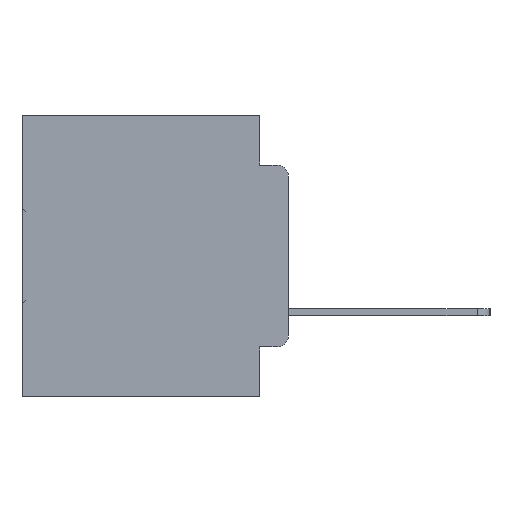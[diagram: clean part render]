
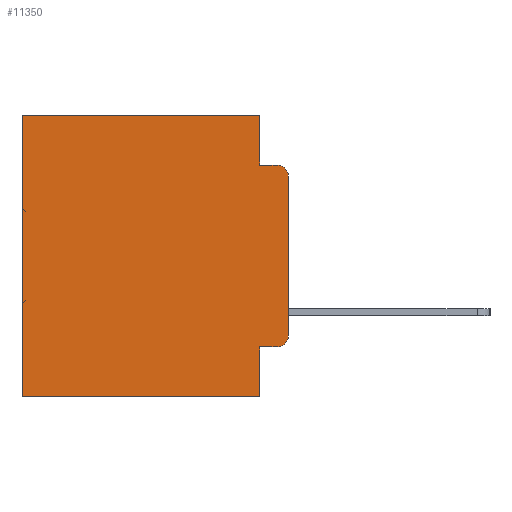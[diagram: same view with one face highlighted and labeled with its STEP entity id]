
A CAD part, left-side view. The second image highlights one B-rep face of the part: STEP entity #11350.
In plain terms, the highlighted planar face has unit normal (-1, 0, 0).
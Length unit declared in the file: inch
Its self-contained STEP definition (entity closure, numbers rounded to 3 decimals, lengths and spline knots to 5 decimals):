
#225 = VERTEX_POINT ( 'NONE', #13336 ) ;
#260 = CARTESIAN_POINT ( 'NONE',  ( 0.298, 0.02, -0.3915 ) ) ;
#282 = CARTESIAN_POINT ( 'NONE',  ( 0.298, 0.051, -0.4115 ) ) ;
#612 = VERTEX_POINT ( 'NONE', #30780 ) ;
#1627 = EDGE_CURVE ( 'NONE', #612, #17676, #18233, .T. ) ;
#1870 = DIRECTION ( 'NONE',  ( 0., -1., 0. ) ) ;
#1932 = CARTESIAN_POINT ( 'NONE',  ( 0.298, 0., 0. ) ) ;
#2597 = LINE ( 'NONE', #282, #29986 ) ;
#2846 = DIRECTION ( 'NONE',  ( 0., 0., -1. ) ) ;
#3049 = VECTOR ( 'NONE', #9485, 39.37008 ) ;
#3264 = LINE ( 'NONE', #29891, #16380 ) ;
#3346 = EDGE_CURVE ( 'NONE', #28680, #26283, #18556, .T. ) ;
#3871 = VECTOR ( 'NONE', #1870, 39.37008 ) ;
#4135 = DIRECTION ( 'NONE',  ( 0., 1., 0. ) ) ;
#4545 = DIRECTION ( 'NONE',  ( 0., 0., -1. ) ) ;
#4864 = VERTEX_POINT ( 'NONE', #20870 ) ;
#5791 = EDGE_CURVE ( 'NONE', #4864, #17000, #7734, .T. ) ;
#6125 = ORIENTED_EDGE ( 'NONE', *, *, #3346, .F. ) ;
#6180 = DIRECTION ( 'NONE',  ( 0., 1., 0. ) ) ;
#6495 = ORIENTED_EDGE ( 'NONE', *, *, #25176, .T. ) ;
#7278 = ORIENTED_EDGE ( 'NONE', *, *, #24792, .F. ) ;
#7734 = LINE ( 'NONE', #29913, #13092 ) ;
#8023 = DIRECTION ( 'NONE',  ( 0., 0., -1. ) ) ;
#8665 = EDGE_CURVE ( 'NONE', #28680, #31448, #2597, .T. ) ;
#9188 = CARTESIAN_POINT ( 'NONE',  ( 0.298, 0.051, 0. ) ) ;
#9239 = LINE ( 'NONE', #24396, #3049 ) ;
#9485 = DIRECTION ( 'NONE',  ( 0., 0., -1. ) ) ;
#10274 = DIRECTION ( 'NONE',  ( -1., 0., 0. ) ) ;
#11350 = ADVANCED_FACE ( 'NONE', ( #23594 ), #17555, .F. ) ;
#12022 = AXIS2_PLACEMENT_3D ( 'NONE', #260, #18476, #2846 ) ;
#12406 = EDGE_CURVE ( 'NONE', #26283, #17676, #3264, .T. ) ;
#12514 = VECTOR ( 'NONE', #6180, 39.37008 ) ;
#13092 = VECTOR ( 'NONE', #22371, 39.37008 ) ;
#13336 = CARTESIAN_POINT ( 'NONE',  ( 0.298, 0.051, -0.0885 ) ) ;
#13847 = ORIENTED_EDGE ( 'NONE', *, *, #23095, .T. ) ;
#13933 = EDGE_CURVE ( 'NONE', #31448, #17000, #23408, .T. ) ;
#14462 = CARTESIAN_POINT ( 'NONE',  ( 0.298, 0.02, -0.4115 ) ) ;
#15552 = ORIENTED_EDGE ( 'NONE', *, *, #8665, .T. ) ;
#16380 = VECTOR ( 'NONE', #4135, 39.37008 ) ;
#17000 = VERTEX_POINT ( 'NONE', #20165 ) ;
#17353 = VERTEX_POINT ( 'NONE', #26588 ) ;
#17500 = VERTEX_POINT ( 'NONE', #24589 ) ;
#17555 = PLANE ( 'NONE',  #24556 ) ;
#17676 = VERTEX_POINT ( 'NONE', #20352 ) ;
#17770 = LINE ( 'NONE', #27684, #3871 ) ;
#18233 = LINE ( 'NONE', #31635, #22556 ) ;
#18476 = DIRECTION ( 'NONE',  ( -1., 0., 0. ) ) ;
#18498 = DIRECTION ( 'NONE',  ( 0., -1., 0. ) ) ;
#18556 = LINE ( 'NONE', #9188, #31191 ) ;
#19328 = LINE ( 'NONE', #21649, #12514 ) ;
#19863 = ORIENTED_EDGE ( 'NONE', *, *, #29887, .F. ) ;
#20085 = DIRECTION ( 'NONE',  ( 1., 0., 0. ) ) ;
#20165 = CARTESIAN_POINT ( 'NONE',  ( 0.298, 0., -0.3915 ) ) ;
#20352 = CARTESIAN_POINT ( 'NONE',  ( 0.298, 0.473, -0.5 ) ) ;
#20361 = ORIENTED_EDGE ( 'NONE', *, *, #13933, .T. ) ;
#20551 = EDGE_LOOP ( 'NONE', ( #30861, #13847, #7278, #19863, #6495, #20680, #25438, #6125, #15552, #20361 ) ) ;
#20680 = ORIENTED_EDGE ( 'NONE', *, *, #1627, .T. ) ;
#20870 = CARTESIAN_POINT ( 'NONE',  ( 0.298, 0., -0.1085 ) ) ;
#21586 = CARTESIAN_POINT ( 'NONE',  ( 0.298, 0.051, -0.5 ) ) ;
#21649 = CARTESIAN_POINT ( 'NONE',  ( 0.298, 0., 0. ) ) ;
#22371 = DIRECTION ( 'NONE',  ( 0., 0., -1. ) ) ;
#22556 = VECTOR ( 'NONE', #27065, 39.37008 ) ;
#23095 = EDGE_CURVE ( 'NONE', #4864, #17500, #29335, .T. ) ;
#23408 = CIRCLE ( 'NONE', #12022, 0.02 ) ;
#23594 = FACE_OUTER_BOUND ( 'NONE', #20551, .T. ) ;
#24396 = CARTESIAN_POINT ( 'NONE',  ( 0.298, 0.051, 0. ) ) ;
#24472 = CARTESIAN_POINT ( 'NONE',  ( 0.298, 0.051, -0.4115 ) ) ;
#24556 = AXIS2_PLACEMENT_3D ( 'NONE', #1932, #20085, #4545 ) ;
#24589 = CARTESIAN_POINT ( 'NONE',  ( 0.298, 0.02, -0.0885 ) ) ;
#24792 = EDGE_CURVE ( 'NONE', #225, #17500, #17770, .T. ) ;
#25176 = EDGE_CURVE ( 'NONE', #17353, #612, #19328, .T. ) ;
#25438 = ORIENTED_EDGE ( 'NONE', *, *, #12406, .F. ) ;
#25558 = CARTESIAN_POINT ( 'NONE',  ( 0.298, 0.02, -0.1085 ) ) ;
#25854 = AXIS2_PLACEMENT_3D ( 'NONE', #25558, #10274, #28140 ) ;
#26283 = VERTEX_POINT ( 'NONE', #21586 ) ;
#26588 = CARTESIAN_POINT ( 'NONE',  ( 0.298, 0.051, 0. ) ) ;
#27065 = DIRECTION ( 'NONE',  ( 0., 0., -1. ) ) ;
#27684 = CARTESIAN_POINT ( 'NONE',  ( 0.298, 0.051, -0.0885 ) ) ;
#28140 = DIRECTION ( 'NONE',  ( 0., 0., -1. ) ) ;
#28680 = VERTEX_POINT ( 'NONE', #24472 ) ;
#29335 = CIRCLE ( 'NONE', #25854, 0.02 ) ;
#29887 = EDGE_CURVE ( 'NONE', #17353, #225, #9239, .T. ) ;
#29891 = CARTESIAN_POINT ( 'NONE',  ( 0.298, 0., -0.5 ) ) ;
#29913 = CARTESIAN_POINT ( 'NONE',  ( 0.298, 0., 0. ) ) ;
#29986 = VECTOR ( 'NONE', #18498, 39.37008 ) ;
#30780 = CARTESIAN_POINT ( 'NONE',  ( 0.298, 0.473, 0. ) ) ;
#30861 = ORIENTED_EDGE ( 'NONE', *, *, #5791, .F. ) ;
#31191 = VECTOR ( 'NONE', #8023, 39.37008 ) ;
#31448 = VERTEX_POINT ( 'NONE', #14462 ) ;
#31635 = CARTESIAN_POINT ( 'NONE',  ( 0.298, 0.473, 0. ) ) ;
